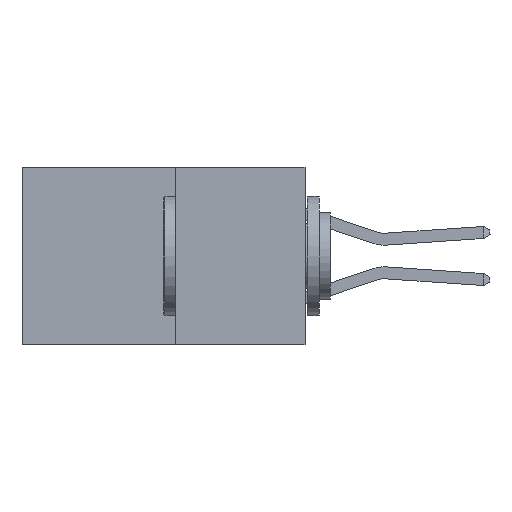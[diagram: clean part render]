
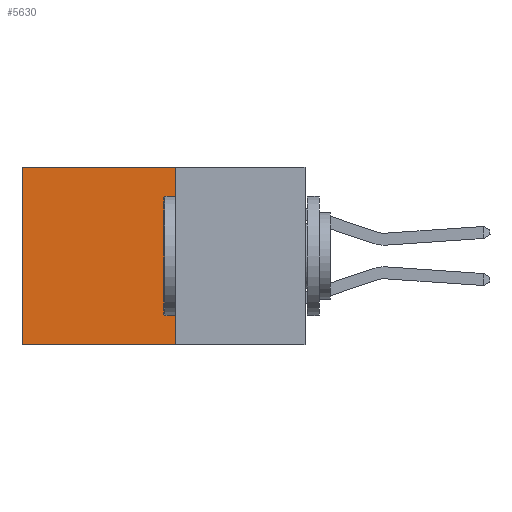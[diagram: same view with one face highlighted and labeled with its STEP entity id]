
A CAD part, left-side view. The second image highlights one B-rep face of the part: STEP entity #5630.
In plain terms, the highlighted planar face has unit normal (-1, 0, 0).
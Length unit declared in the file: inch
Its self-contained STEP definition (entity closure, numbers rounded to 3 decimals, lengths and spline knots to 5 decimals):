
#848 = VECTOR ( 'NONE', #13957, 39.37008 ) ;
#1514 = LINE ( 'NONE', #11733, #848 ) ;
#3183 = CARTESIAN_POINT ( 'NONE',  ( 0.277, 0.27, -0.37 ) ) ;
#3941 = EDGE_LOOP ( 'NONE', ( #5722, #23824, #12965, #19433 ) ) ;
#4877 = EDGE_CURVE ( 'NONE', #21088, #10443, #21340, .T. ) ;
#5630 = ADVANCED_FACE ( 'NONE', ( #17584 ), #23491, .F. ) ;
#5722 = ORIENTED_EDGE ( 'NONE', *, *, #5796, .T. ) ;
#5796 = EDGE_CURVE ( 'NONE', #10443, #20981, #19250, .T. ) ;
#8920 = EDGE_CURVE ( 'NONE', #15276, #20981, #20336, .T. ) ;
#10443 = VERTEX_POINT ( 'NONE', #20508 ) ;
#11004 = CARTESIAN_POINT ( 'NONE',  ( 0.277, 0.27, 0. ) ) ;
#11065 = CARTESIAN_POINT ( 'NONE',  ( 0.277, 0.27, -0.37 ) ) ;
#11733 = CARTESIAN_POINT ( 'NONE',  ( 0.277, 0.27, -0.37 ) ) ;
#12965 = ORIENTED_EDGE ( 'NONE', *, *, #25907, .F. ) ;
#13957 = DIRECTION ( 'NONE',  ( 0., 0., -1. ) ) ;
#14577 = VECTOR ( 'NONE', #24090, 39.37008 ) ;
#15276 = VERTEX_POINT ( 'NONE', #3183 ) ;
#16348 = DIRECTION ( 'NONE',  ( 0., 1., 0. ) ) ;
#17203 = CARTESIAN_POINT ( 'NONE',  ( 0.277, 0.27, 0. ) ) ;
#17584 = FACE_OUTER_BOUND ( 'NONE', #3941, .T. ) ;
#18577 = VECTOR ( 'NONE', #25255, 39.37008 ) ;
#19250 = LINE ( 'NONE', #27888, #18577 ) ;
#19433 = ORIENTED_EDGE ( 'NONE', *, *, #4877, .T. ) ;
#20336 = LINE ( 'NONE', #11065, #14577 ) ;
#20508 = CARTESIAN_POINT ( 'NONE',  ( 0.277, 0.59, 0. ) ) ;
#20685 = VECTOR ( 'NONE', #16348, 39.37008 ) ;
#20981 = VERTEX_POINT ( 'NONE', #25716 ) ;
#21088 = VERTEX_POINT ( 'NONE', #11004 ) ;
#21126 = DIRECTION ( 'NONE',  ( 0., 0., -1. ) ) ;
#21340 = LINE ( 'NONE', #17203, #20685 ) ;
#21525 = DIRECTION ( 'NONE',  ( 1., 0., 0. ) ) ;
#21554 = CARTESIAN_POINT ( 'NONE',  ( 0.277, 0.27, -0.37 ) ) ;
#21940 = AXIS2_PLACEMENT_3D ( 'NONE', #21554, #21525, #21126 ) ;
#23491 = PLANE ( 'NONE',  #21940 ) ;
#23824 = ORIENTED_EDGE ( 'NONE', *, *, #8920, .F. ) ;
#24090 = DIRECTION ( 'NONE',  ( 0., 1., 0. ) ) ;
#25255 = DIRECTION ( 'NONE',  ( 0., 0., -1. ) ) ;
#25716 = CARTESIAN_POINT ( 'NONE',  ( 0.277, 0.59, -0.37 ) ) ;
#25907 = EDGE_CURVE ( 'NONE', #21088, #15276, #1514, .T. ) ;
#27888 = CARTESIAN_POINT ( 'NONE',  ( 0.277, 0.59, -0.37 ) ) ;
